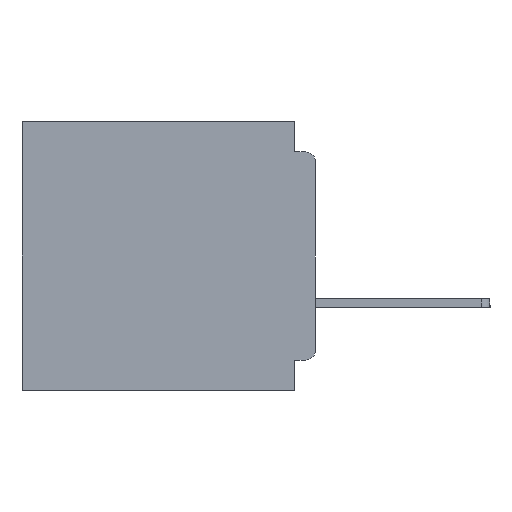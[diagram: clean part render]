
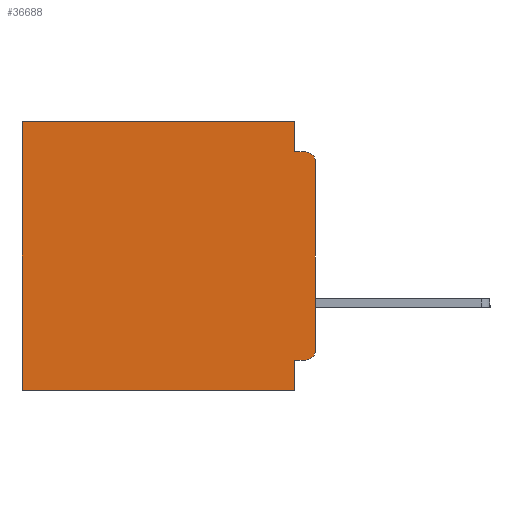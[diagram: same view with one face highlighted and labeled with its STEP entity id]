
A CAD part, left-side view. The second image highlights one B-rep face of the part: STEP entity #36688.
In plain terms, the highlighted planar face has unit normal (-1, 0, 0).
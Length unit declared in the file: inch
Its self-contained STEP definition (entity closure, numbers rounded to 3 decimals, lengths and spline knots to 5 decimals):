
#1297 = ORIENTED_EDGE ( 'NONE', *, *, #12067, .F. ) ;
#1337 = CARTESIAN_POINT ( 'NONE',  ( 0.3, 0.031, -0.4 ) ) ;
#1666 = VECTOR ( 'NONE', #33478, 39.37008 ) ;
#3207 = CARTESIAN_POINT ( 'NONE',  ( 0.3, 0.015, -0.045 ) ) ;
#3378 = DIRECTION ( 'NONE',  ( 1., 0., 0. ) ) ;
#3808 = VECTOR ( 'NONE', #45078, 39.37008 ) ;
#4496 = VECTOR ( 'NONE', #6786, 39.37008 ) ;
#4545 = CARTESIAN_POINT ( 'NONE',  ( 0.3, 0.015, -0.355 ) ) ;
#4617 = CARTESIAN_POINT ( 'NONE',  ( 0.3, 0.031, -0.045 ) ) ;
#5181 = ORIENTED_EDGE ( 'NONE', *, *, #26343, .T. ) ;
#5753 = LINE ( 'NONE', #43080, #4496 ) ;
#5999 = EDGE_CURVE ( 'NONE', #39396, #30515, #19084, .T. ) ;
#6786 = DIRECTION ( 'NONE',  ( 0., 1., 0. ) ) ;
#7131 = CARTESIAN_POINT ( 'NONE',  ( 0.3, 0.015, -0.34 ) ) ;
#7691 = DIRECTION ( 'NONE',  ( 0., 0., -1. ) ) ;
#7739 = LINE ( 'NONE', #22400, #17241 ) ;
#8110 = AXIS2_PLACEMENT_3D ( 'NONE', #7131, #35471, #11213 ) ;
#8282 = VERTEX_POINT ( 'NONE', #39835 ) ;
#8505 = LINE ( 'NONE', #10107, #50231 ) ;
#8776 = EDGE_CURVE ( 'NONE', #8282, #34374, #15831, .T. ) ;
#10107 = CARTESIAN_POINT ( 'NONE',  ( 0.3, 0., 0. ) ) ;
#10200 = ORIENTED_EDGE ( 'NONE', *, *, #44764, .F. ) ;
#10795 = CARTESIAN_POINT ( 'NONE',  ( 0.3, 0., -0.045 ) ) ;
#11213 = DIRECTION ( 'NONE',  ( 0., 0., -1. ) ) ;
#11814 = EDGE_CURVE ( 'NONE', #35631, #33645, #12405, .T. ) ;
#12067 = EDGE_CURVE ( 'NONE', #30515, #34374, #34580, .T. ) ;
#12405 = LINE ( 'NONE', #21277, #1666 ) ;
#12705 = ORIENTED_EDGE ( 'NONE', *, *, #33774, .F. ) ;
#13031 = VECTOR ( 'NONE', #26914, 39.37008 ) ;
#13486 = VERTEX_POINT ( 'NONE', #27144 ) ;
#14416 = EDGE_CURVE ( 'NONE', #8282, #13486, #19683, .T. ) ;
#14835 = CARTESIAN_POINT ( 'NONE',  ( 0.3, 0.015, -0.06 ) ) ;
#15023 = CARTESIAN_POINT ( 'NONE',  ( 0.3, 0.031, 0. ) ) ;
#15831 = CIRCLE ( 'NONE', #33624, 0.015 ) ;
#16630 = EDGE_CURVE ( 'NONE', #46209, #32738, #18781, .T. ) ;
#16754 = EDGE_LOOP ( 'NONE', ( #37999, #28523, #1297, #45590, #27903, #32981, #12705, #10200, #34962, #5181 ) ) ;
#17241 = VECTOR ( 'NONE', #42578, 39.37008 ) ;
#17484 = VECTOR ( 'NONE', #25753, 39.37008 ) ;
#17665 = AXIS2_PLACEMENT_3D ( 'NONE', #27645, #3378, #31713 ) ;
#18538 = CARTESIAN_POINT ( 'NONE',  ( 0.3, 0.437, 0. ) ) ;
#18781 = LINE ( 'NONE', #21474, #17484 ) ;
#18909 = DIRECTION ( 'NONE',  ( 0., 0., -1. ) ) ;
#19084 = LINE ( 'NONE', #27887, #51272 ) ;
#19683 = LINE ( 'NONE', #41013, #3808 ) ;
#21277 = CARTESIAN_POINT ( 'NONE',  ( 0.3, 0., -0.355 ) ) ;
#21474 = CARTESIAN_POINT ( 'NONE',  ( 0.3, 0.437, -0.4 ) ) ;
#22400 = CARTESIAN_POINT ( 'NONE',  ( 0.3, 0.031, -0.4 ) ) ;
#25753 = DIRECTION ( 'NONE',  ( 0., 0., -1. ) ) ;
#26279 = CARTESIAN_POINT ( 'NONE',  ( 0.3, 0.031, -0.355 ) ) ;
#26343 = EDGE_CURVE ( 'NONE', #35631, #13486, #46329, .T. ) ;
#26914 = DIRECTION ( 'NONE',  ( 0., -1., 0. ) ) ;
#27144 = CARTESIAN_POINT ( 'NONE',  ( 0.3, 0., -0.34 ) ) ;
#27645 = CARTESIAN_POINT ( 'NONE',  ( 0.3, 0., -0.4 ) ) ;
#27887 = CARTESIAN_POINT ( 'NONE',  ( 0.3, 0.031, 0. ) ) ;
#27903 = ORIENTED_EDGE ( 'NONE', *, *, #43687, .T. ) ;
#28523 = ORIENTED_EDGE ( 'NONE', *, *, #8776, .T. ) ;
#28675 = CARTESIAN_POINT ( 'NONE',  ( 0.3, 0.437, -0.4 ) ) ;
#30515 = VERTEX_POINT ( 'NONE', #4617 ) ;
#31713 = DIRECTION ( 'NONE',  ( 0., 0., -1. ) ) ;
#32738 = VERTEX_POINT ( 'NONE', #28675 ) ;
#32981 = ORIENTED_EDGE ( 'NONE', *, *, #16630, .T. ) ;
#33478 = DIRECTION ( 'NONE',  ( 0., 1., 0. ) ) ;
#33624 = AXIS2_PLACEMENT_3D ( 'NONE', #14835, #43152, #18909 ) ;
#33645 = VERTEX_POINT ( 'NONE', #26279 ) ;
#33774 = EDGE_CURVE ( 'NONE', #42297, #32738, #5753, .T. ) ;
#34374 = VERTEX_POINT ( 'NONE', #3207 ) ;
#34580 = LINE ( 'NONE', #10795, #13031 ) ;
#34962 = ORIENTED_EDGE ( 'NONE', *, *, #11814, .F. ) ;
#35471 = DIRECTION ( 'NONE',  ( -1., 0., 0. ) ) ;
#35631 = VERTEX_POINT ( 'NONE', #4545 ) ;
#36688 = ADVANCED_FACE ( 'NONE', ( #47892 ), #47774, .F. ) ;
#37999 = ORIENTED_EDGE ( 'NONE', *, *, #14416, .F. ) ;
#39396 = VERTEX_POINT ( 'NONE', #15023 ) ;
#39835 = CARTESIAN_POINT ( 'NONE',  ( 0.3, 0., -0.06 ) ) ;
#41013 = CARTESIAN_POINT ( 'NONE',  ( 0.3, 0., -0.4 ) ) ;
#42297 = VERTEX_POINT ( 'NONE', #1337 ) ;
#42578 = DIRECTION ( 'NONE',  ( 0., 0., -1. ) ) ;
#43080 = CARTESIAN_POINT ( 'NONE',  ( 0.3, 0., -0.4 ) ) ;
#43152 = DIRECTION ( 'NONE',  ( -1., 0., 0. ) ) ;
#43687 = EDGE_CURVE ( 'NONE', #39396, #46209, #8505, .T. ) ;
#44764 = EDGE_CURVE ( 'NONE', #33645, #42297, #7739, .T. ) ;
#45078 = DIRECTION ( 'NONE',  ( 0., 0., -1. ) ) ;
#45590 = ORIENTED_EDGE ( 'NONE', *, *, #5999, .F. ) ;
#46209 = VERTEX_POINT ( 'NONE', #18538 ) ;
#46329 = CIRCLE ( 'NONE', #8110, 0.015 ) ;
#47774 = PLANE ( 'NONE',  #17665 ) ;
#47892 = FACE_OUTER_BOUND ( 'NONE', #16754, .T. ) ;
#50231 = VECTOR ( 'NONE', #50753, 39.37008 ) ;
#50753 = DIRECTION ( 'NONE',  ( 0., 1., 0. ) ) ;
#51272 = VECTOR ( 'NONE', #7691, 39.37008 ) ;
